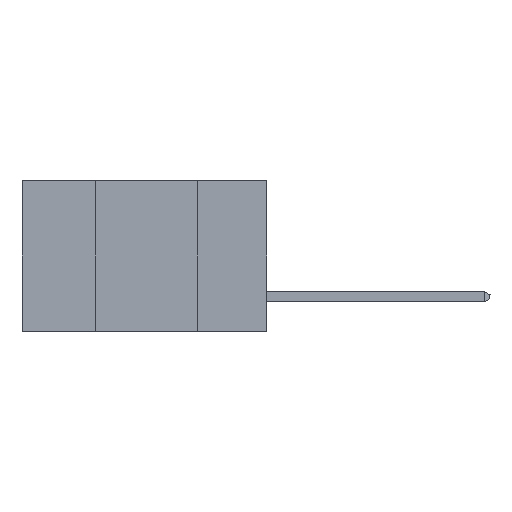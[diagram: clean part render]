
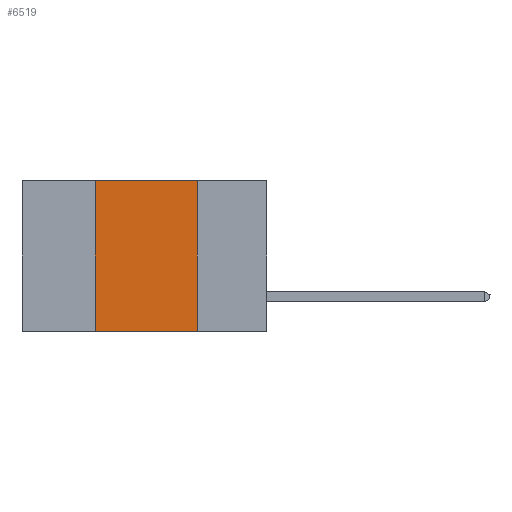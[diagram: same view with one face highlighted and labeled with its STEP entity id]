
A CAD part, left-side view. The second image highlights one B-rep face of the part: STEP entity #6519.
In plain terms, the highlighted planar face has unit normal (-1, 0, 0).
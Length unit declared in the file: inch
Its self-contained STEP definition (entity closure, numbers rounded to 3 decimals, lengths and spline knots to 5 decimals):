
#1208 = VERTEX_POINT ( 'NONE', #8242 ) ;
#4187 = CARTESIAN_POINT ( 'NONE',  ( 0., 0.17, -0.37 ) ) ;
#5244 = DIRECTION ( 'NONE',  ( 0., -1., 0. ) ) ;
#5559 = CARTESIAN_POINT ( 'NONE',  ( 0., 0.6, 0. ) ) ;
#6519 = ADVANCED_FACE ( 'NONE', ( #17500 ), #15090, .F. ) ;
#8242 = CARTESIAN_POINT ( 'NONE',  ( 0., 0.42, 0. ) ) ;
#8715 = LINE ( 'NONE', #10545, #14687 ) ;
#10047 = DIRECTION ( 'NONE',  ( 0., 0., 1. ) ) ;
#10545 = CARTESIAN_POINT ( 'NONE',  ( 0., 0.17, 0. ) ) ;
#12114 = EDGE_CURVE ( 'NONE', #1208, #12647, #22756, .T. ) ;
#12285 = CARTESIAN_POINT ( 'NONE',  ( 0., 0.6, -0.37 ) ) ;
#12647 = VERTEX_POINT ( 'NONE', #13718 ) ;
#12779 = DIRECTION ( 'NONE',  ( 0., 0., -1. ) ) ;
#13153 = VECTOR ( 'NONE', #27168, 39.37008 ) ;
#13718 = CARTESIAN_POINT ( 'NONE',  ( 0., 0.17, 0. ) ) ;
#14065 = VECTOR ( 'NONE', #5244, 39.37008 ) ;
#14254 = VERTEX_POINT ( 'NONE', #17290 ) ;
#14289 = EDGE_CURVE ( 'NONE', #12647, #17834, #8715, .T. ) ;
#14687 = VECTOR ( 'NONE', #24899, 39.37008 ) ;
#15090 = PLANE ( 'NONE',  #28777 ) ;
#15386 = EDGE_LOOP ( 'NONE', ( #29575, #21474, #27898, #22202 ) ) ;
#16974 = EDGE_CURVE ( 'NONE', #14254, #17834, #29404, .T. ) ;
#17290 = CARTESIAN_POINT ( 'NONE',  ( 0., 0.42, -0.37 ) ) ;
#17500 = FACE_OUTER_BOUND ( 'NONE', #15386, .T. ) ;
#17834 = VERTEX_POINT ( 'NONE', #4187 ) ;
#17940 = LINE ( 'NONE', #24806, #29273 ) ;
#21474 = ORIENTED_EDGE ( 'NONE', *, *, #12114, .F. ) ;
#22202 = ORIENTED_EDGE ( 'NONE', *, *, #16974, .T. ) ;
#22756 = LINE ( 'NONE', #29166, #14065 ) ;
#24806 = CARTESIAN_POINT ( 'NONE',  ( 0., 0.42, 0. ) ) ;
#24899 = DIRECTION ( 'NONE',  ( 0., 0., -1. ) ) ;
#27168 = DIRECTION ( 'NONE',  ( 0., -1., 0. ) ) ;
#27244 = DIRECTION ( 'NONE',  ( 1., 0., 0. ) ) ;
#27855 = EDGE_CURVE ( 'NONE', #14254, #1208, #17940, .T. ) ;
#27898 = ORIENTED_EDGE ( 'NONE', *, *, #27855, .F. ) ;
#28777 = AXIS2_PLACEMENT_3D ( 'NONE', #5559, #27244, #12779 ) ;
#29166 = CARTESIAN_POINT ( 'NONE',  ( 0., 0.6, 0. ) ) ;
#29273 = VECTOR ( 'NONE', #10047, 39.37008 ) ;
#29404 = LINE ( 'NONE', #12285, #13153 ) ;
#29575 = ORIENTED_EDGE ( 'NONE', *, *, #14289, .F. ) ;
